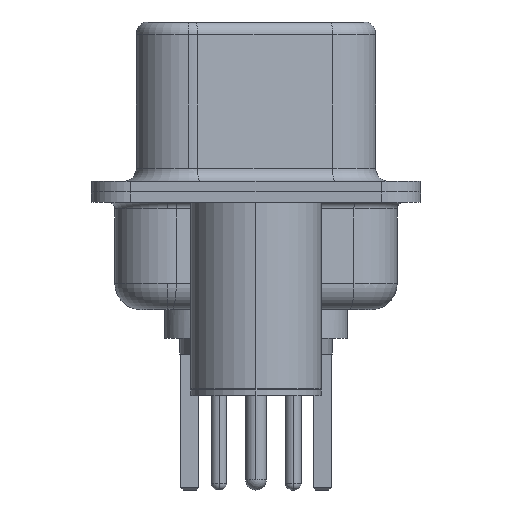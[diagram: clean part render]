
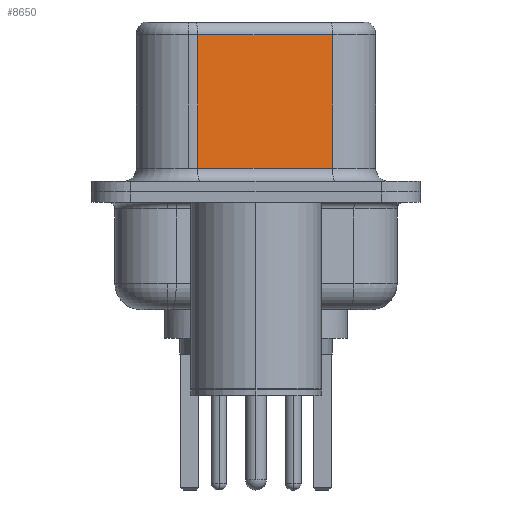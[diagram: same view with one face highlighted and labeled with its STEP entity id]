
A CAD part, left-side view. The second image highlights one B-rep face of the part: STEP entity #8650.
In plain terms, the highlighted planar face has unit normal (-0.985, -0.174, 0).
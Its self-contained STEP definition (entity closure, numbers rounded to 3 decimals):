
#624 = CARTESIAN_POINT ( 'NONE',  ( 3.655, 2.233, 0.9 ) ) ;
#952 = PLANE ( 'NONE',  #2110 ) ;
#1145 = CARTESIAN_POINT ( 'NONE',  ( 4.565, -2.927, 0.9 ) ) ;
#2029 = VERTEX_POINT ( 'NONE', #624 ) ;
#2110 = AXIS2_PLACEMENT_3D ( 'NONE', #12045, #2463, #13654 ) ;
#2463 = DIRECTION ( 'NONE',  ( 0.985, 0.174, 0. ) ) ;
#2520 = VECTOR ( 'NONE', #14655, 1000. ) ;
#2988 = CARTESIAN_POINT ( 'NONE',  ( 4.565, -2.927, 6.02 ) ) ;
#3127 = ORIENTED_EDGE ( 'NONE', *, *, #12889, .T. ) ;
#3592 = ORIENTED_EDGE ( 'NONE', *, *, #15558, .T. ) ;
#5017 = ORIENTED_EDGE ( 'NONE', *, *, #14278, .F. ) ;
#6026 = DIRECTION ( 'NONE',  ( 0., 0., -1. ) ) ;
#6772 = VECTOR ( 'NONE', #6026, 1000. ) ;
#6953 = EDGE_LOOP ( 'NONE', ( #5017, #3127, #3592, #11851 ) ) ;
#7046 = VECTOR ( 'NONE', #12548, 1000. ) ;
#7265 = LINE ( 'NONE', #12492, #6772 ) ;
#7679 = CARTESIAN_POINT ( 'NONE',  ( 4.565, -2.927, 0.9 ) ) ;
#8650 = ADVANCED_FACE ( 'NONE', ( #14488 ), #952, .F. ) ;
#8739 = VERTEX_POINT ( 'NONE', #1145 ) ;
#9306 = DIRECTION ( 'NONE',  ( 0.174, -0.985, 0. ) ) ;
#11118 = LINE ( 'NONE', #7679, #18928 ) ;
#11394 = LINE ( 'NONE', #2988, #7046 ) ;
#11851 = ORIENTED_EDGE ( 'NONE', *, *, #14282, .T. ) ;
#12045 = CARTESIAN_POINT ( 'NONE',  ( 4.565, -2.927, 6.52 ) ) ;
#12492 = CARTESIAN_POINT ( 'NONE',  ( 4.565, -2.927, 6.52 ) ) ;
#12548 = DIRECTION ( 'NONE',  ( -0.174, 0.985, 0. ) ) ;
#12889 = EDGE_CURVE ( 'NONE', #16991, #16353, #11394, .T. ) ;
#13022 = CARTESIAN_POINT ( 'NONE',  ( 3.655, 2.233, 6.52 ) ) ;
#13654 = DIRECTION ( 'NONE',  ( -0.174, 0.985, 0. ) ) ;
#14278 = EDGE_CURVE ( 'NONE', #16991, #8739, #7265, .T. ) ;
#14282 = EDGE_CURVE ( 'NONE', #2029, #8739, #11118, .T. ) ;
#14488 = FACE_OUTER_BOUND ( 'NONE', #6953, .T. ) ;
#14655 = DIRECTION ( 'NONE',  ( 0., 0., -1. ) ) ;
#15310 = LINE ( 'NONE', #13022, #2520 ) ;
#15558 = EDGE_CURVE ( 'NONE', #16353, #2029, #15310, .T. ) ;
#16353 = VERTEX_POINT ( 'NONE', #19679 ) ;
#16991 = VERTEX_POINT ( 'NONE', #19205 ) ;
#18928 = VECTOR ( 'NONE', #9306, 1000. ) ;
#19205 = CARTESIAN_POINT ( 'NONE',  ( 4.565, -2.927, 6.02 ) ) ;
#19679 = CARTESIAN_POINT ( 'NONE',  ( 3.655, 2.233, 6.02 ) ) ;
